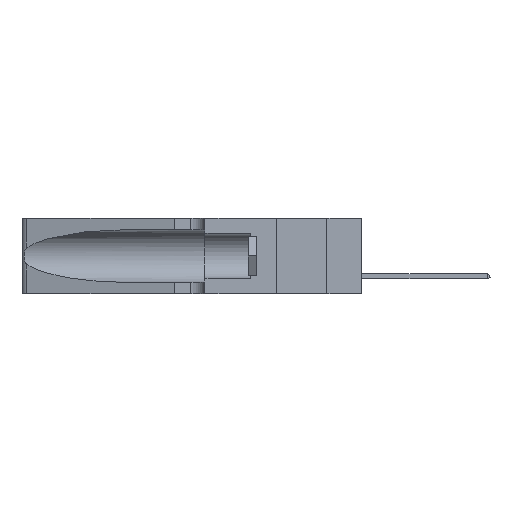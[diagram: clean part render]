
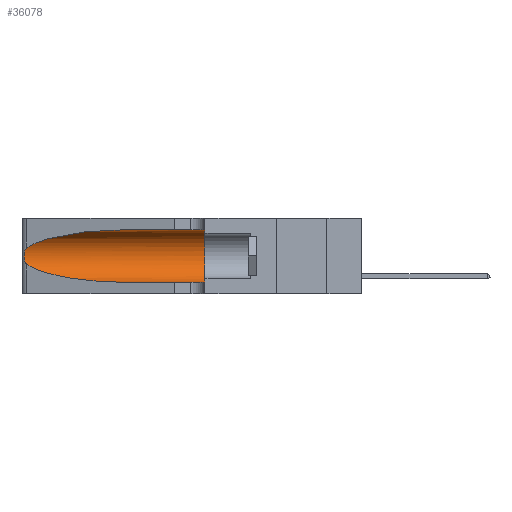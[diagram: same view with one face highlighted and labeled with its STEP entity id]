
A CAD part, left-side view. The second image highlights one B-rep face of the part: STEP entity #36078.
In plain terms, the highlighted cylindrical face has radius 3.308 mm (diameter 6.617 mm), a partial arc.
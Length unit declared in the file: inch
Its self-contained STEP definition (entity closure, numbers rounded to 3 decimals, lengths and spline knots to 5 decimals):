
#1231 = CARTESIAN_POINT ( 'NONE',  ( 0.1305, 0.72297, 0.31525 ) ) ;
#1482 = CARTESIAN_POINT ( 'NONE',  ( 0.25487, 1.22718, 0.14631 ) ) ;
#1866 = B_SPLINE_CURVE_WITH_KNOTS ( 'NONE', 3,
 ( #9046, #28339, #34820, #15440, #29604, #16287, #10474, #13992, #17260, #39328, #36350, #27168, #23885, #1482 ),
 .UNSPECIFIED., .F., .F.,
 ( 4, 2, 2, 2, 2, 2, 4 ),
 ( 0., 0.00027, 0.00053, 0.00107, 0.0016, 0.00187, 0.00214 ),
 .UNSPECIFIED. ) ;
#2469 = AXIS2_PLACEMENT_3D ( 'NONE', #41863, #18852, #28922 ) ;
#3973 = CARTESIAN_POINT ( 'NONE',  ( 0.2373, 1.15595, 0.28018 ) ) ;
#4383 = EDGE_CURVE ( 'NONE', #10153, #15193, #1866, .T. ) ;
#4906 = VECTOR ( 'NONE', #15864, 39.37008 ) ;
#5334 = EDGE_CURVE ( 'NONE', #5819, #18060, #21758, .T. ) ;
#5819 = VERTEX_POINT ( 'NONE', #35287 ) ;
#5871 = DIRECTION ( 'NONE',  ( 0., -1., 0. ) ) ;
#6226 = CARTESIAN_POINT ( 'NONE',  ( 0.2373, 1.15595, 0.08982 ) ) ;
#6293 = DIRECTION ( 'NONE',  ( 0., -1., 0. ) ) ;
#8131 =( BOUNDED_CURVE ( )  B_SPLINE_CURVE ( 3, ( #34567, #6226, #10209, #23094 ),
 .UNSPECIFIED., .F., .F. ) 
 B_SPLINE_CURVE_WITH_KNOTS ( ( 4, 4 ),
 ( 3.44316, 4.71239 ),
 .UNSPECIFIED. ) 
 CURVE ( )  GEOMETRIC_REPRESENTATION_ITEM ( )  RATIONAL_B_SPLINE_CURVE ( ( 1., 0.87, 0.87, 1. ) ) 
 REPRESENTATION_ITEM ( '' )  );
#9046 = CARTESIAN_POINT ( 'NONE',  ( 0.25487, 1.22718, 0.22369 ) ) ;
#9420 = DIRECTION ( 'NONE',  ( 0., 0., -1. ) ) ;
#10153 = VERTEX_POINT ( 'NONE', #34515 ) ;
#10209 = CARTESIAN_POINT ( 'NONE',  ( 0.18966, 0.96281, 0.05475 ) ) ;
#10474 = CARTESIAN_POINT ( 'NONE',  ( 0.26075, 1.23896, 0.19203 ) ) ;
#10483 = FACE_OUTER_BOUND ( 'NONE', #40292, .T. ) ;
#13117 = EDGE_CURVE ( 'NONE', #15193, #28830, #8131, .T. ) ;
#13506 = CYLINDRICAL_SURFACE ( 'NONE', #17433, 0.13025 ) ;
#13992 = CARTESIAN_POINT ( 'NONE',  ( 0.26075, 1.23896, 0.178 ) ) ;
#14827 = CARTESIAN_POINT ( 'NONE',  ( 0.1305, 0.35, 0.05475 ) ) ;
#14866 = VECTOR ( 'NONE', #5871, 39.37008 ) ;
#15193 = VERTEX_POINT ( 'NONE', #29534 ) ;
#15406 = ORIENTED_EDGE ( 'NONE', *, *, #35373, .T. ) ;
#15440 = CARTESIAN_POINT ( 'NONE',  ( 0.25787, 1.23484, 0.2124 ) ) ;
#15864 = DIRECTION ( 'NONE',  ( 0., -1., 0. ) ) ;
#16287 = CARTESIAN_POINT ( 'NONE',  ( 0.26018, 1.23835, 0.19895 ) ) ;
#17260 = CARTESIAN_POINT ( 'NONE',  ( 0.26017, 1.23833, 0.17102 ) ) ;
#17433 = AXIS2_PLACEMENT_3D ( 'NONE', #35181, #6293, #9420 ) ;
#18060 = VERTEX_POINT ( 'NONE', #14827 ) ;
#18410 = LINE ( 'NONE', #41255, #14866 ) ;
#18620 = ORIENTED_EDGE ( 'NONE', *, *, #20250, .T. ) ;
#18852 = DIRECTION ( 'NONE',  ( 0., 1., 0. ) ) ;
#19834 = CARTESIAN_POINT ( 'NONE',  ( 0.1305, 0.72297, 0.31525 ) ) ;
#20250 = EDGE_CURVE ( 'NONE', #26667, #10153, #27646, .T. ) ;
#21164 = LINE ( 'NONE', #21975, #4906 ) ;
#21758 = CIRCLE ( 'NONE', #2469, 0.13025 ) ;
#21975 = CARTESIAN_POINT ( 'NONE',  ( 0.1305, 1.61858, 0.05475 ) ) ;
#23094 = CARTESIAN_POINT ( 'NONE',  ( 0.1305, 0.72297, 0.05475 ) ) ;
#23715 = ORIENTED_EDGE ( 'NONE', *, *, #13117, .T. ) ;
#23885 = CARTESIAN_POINT ( 'NONE',  ( 0.25555, 1.22993, 0.14849 ) ) ;
#25487 = ORIENTED_EDGE ( 'NONE', *, *, #5334, .F. ) ;
#26667 = VERTEX_POINT ( 'NONE', #1231 ) ;
#27168 = CARTESIAN_POINT ( 'NONE',  ( 0.25639, 1.23186, 0.15144 ) ) ;
#27277 = ORIENTED_EDGE ( 'NONE', *, *, #37460, .F. ) ;
#27646 =( BOUNDED_CURVE ( )  B_SPLINE_CURVE ( 3, ( #19834, #30596, #3973, #34975 ),
 .UNSPECIFIED., .F., .F. ) 
 B_SPLINE_CURVE_WITH_KNOTS ( ( 4, 4 ),
 ( 1.5708, 2.84003 ),
 .UNSPECIFIED. ) 
 CURVE ( )  GEOMETRIC_REPRESENTATION_ITEM ( )  RATIONAL_B_SPLINE_CURVE ( ( 1., 0.87, 0.87, 1. ) ) 
 REPRESENTATION_ITEM ( '' )  );
#28339 = CARTESIAN_POINT ( 'NONE',  ( 0.25555, 1.22994, 0.2215 ) ) ;
#28664 = CARTESIAN_POINT ( 'NONE',  ( 0.1305, 0.72297, 0.05475 ) ) ;
#28830 = VERTEX_POINT ( 'NONE', #28664 ) ;
#28922 = DIRECTION ( 'NONE',  ( 0., 0., 1. ) ) ;
#29534 = CARTESIAN_POINT ( 'NONE',  ( 0.25487, 1.22718, 0.14631 ) ) ;
#29604 = CARTESIAN_POINT ( 'NONE',  ( 0.25854, 1.2359, 0.20912 ) ) ;
#29892 = ORIENTED_EDGE ( 'NONE', *, *, #4383, .T. ) ;
#30596 = CARTESIAN_POINT ( 'NONE',  ( 0.18966, 0.96281, 0.31525 ) ) ;
#34515 = CARTESIAN_POINT ( 'NONE',  ( 0.25487, 1.22718, 0.22369 ) ) ;
#34567 = CARTESIAN_POINT ( 'NONE',  ( 0.25487, 1.22718, 0.14631 ) ) ;
#34820 = CARTESIAN_POINT ( 'NONE',  ( 0.25639, 1.23184, 0.21858 ) ) ;
#34975 = CARTESIAN_POINT ( 'NONE',  ( 0.25487, 1.22718, 0.22369 ) ) ;
#35181 = CARTESIAN_POINT ( 'NONE',  ( 0.1305, 1.61858, 0.185 ) ) ;
#35287 = CARTESIAN_POINT ( 'NONE',  ( 0.1305, 0.35, 0.31525 ) ) ;
#35373 = EDGE_CURVE ( 'NONE', #28830, #18060, #21164, .T. ) ;
#36078 = ADVANCED_FACE ( 'NONE', ( #10483 ), #13506, .F. ) ;
#36350 = CARTESIAN_POINT ( 'NONE',  ( 0.25789, 1.23486, 0.15765 ) ) ;
#37460 = EDGE_CURVE ( 'NONE', #26667, #5819, #18410, .T. ) ;
#39328 = CARTESIAN_POINT ( 'NONE',  ( 0.25856, 1.23593, 0.16098 ) ) ;
#40292 = EDGE_LOOP ( 'NONE', ( #18620, #29892, #23715, #15406, #25487, #27277 ) ) ;
#41255 = CARTESIAN_POINT ( 'NONE',  ( 0.1305, 1.61858, 0.31525 ) ) ;
#41863 = CARTESIAN_POINT ( 'NONE',  ( 0.1305, 0.35, 0.185 ) ) ;
